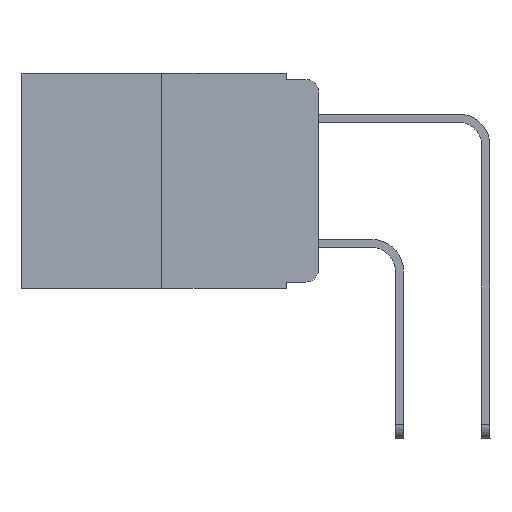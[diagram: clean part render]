
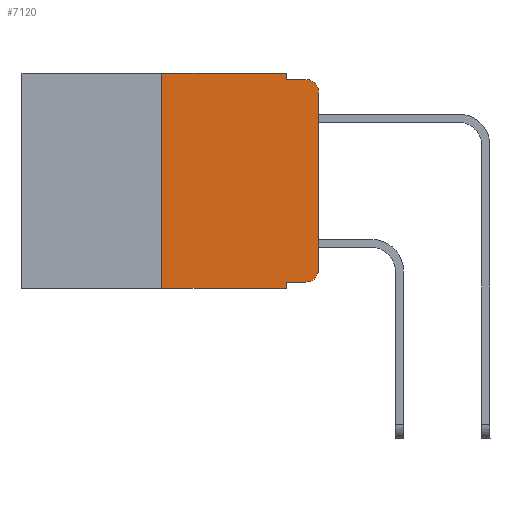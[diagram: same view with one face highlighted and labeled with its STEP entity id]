
A CAD part, left-side view. The second image highlights one B-rep face of the part: STEP entity #7120.
In plain terms, the highlighted planar face has unit normal (-1, 0, 0).
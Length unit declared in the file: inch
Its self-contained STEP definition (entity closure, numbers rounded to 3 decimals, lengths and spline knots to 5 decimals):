
#193 = CARTESIAN_POINT ( 'NONE',  ( 0., 0.473, 0. ) ) ;
#312 = VERTEX_POINT ( 'NONE', #9837 ) ;
#539 = ORIENTED_EDGE ( 'NONE', *, *, #7742, .F. ) ;
#586 = VECTOR ( 'NONE', #9702, 39.37008 ) ;
#711 = CARTESIAN_POINT ( 'NONE',  ( 0., 0.25, -0.343 ) ) ;
#845 = DIRECTION ( 'NONE',  ( 0., 0., -1. ) ) ;
#947 = LINE ( 'NONE', #4866, #586 ) ;
#954 = EDGE_CURVE ( 'NONE', #5619, #1079, #7166, .T. ) ;
#1079 = VERTEX_POINT ( 'NONE', #5046 ) ;
#1091 = EDGE_CURVE ( 'NONE', #1547, #6179, #9170, .T. ) ;
#1263 = CARTESIAN_POINT ( 'NONE',  ( 0., 0.051, -0.343 ) ) ;
#1268 = CARTESIAN_POINT ( 'NONE',  ( 0., 0.02, -0.313 ) ) ;
#1378 = EDGE_CURVE ( 'NONE', #1547, #5619, #9984, .T. ) ;
#1421 = ORIENTED_EDGE ( 'NONE', *, *, #8279, .F. ) ;
#1547 = VERTEX_POINT ( 'NONE', #9796 ) ;
#2402 = CARTESIAN_POINT ( 'NONE',  ( 0., 0.473, 0. ) ) ;
#2510 = VECTOR ( 'NONE', #5384, 39.37008 ) ;
#2611 = VECTOR ( 'NONE', #11231, 39.37008 ) ;
#2626 = AXIS2_PLACEMENT_3D ( 'NONE', #1268, #9910, #845 ) ;
#2719 = AXIS2_PLACEMENT_3D ( 'NONE', #193, #10028, #5282 ) ;
#2840 = DIRECTION ( 'NONE',  ( 0., -1., 0. ) ) ;
#2870 = VERTEX_POINT ( 'NONE', #3173 ) ;
#2975 = VECTOR ( 'NONE', #2840, 39.37008 ) ;
#3173 = CARTESIAN_POINT ( 'NONE',  ( 0., 0.051, 0. ) ) ;
#3471 = VECTOR ( 'NONE', #6111, 39.37008 ) ;
#3953 = ORIENTED_EDGE ( 'NONE', *, *, #1091, .F. ) ;
#4580 = EDGE_LOOP ( 'NONE', ( #8659, #5937, #6307, #1421, #7128, #539, #10409, #3953, #6541, #10649 ) ) ;
#4604 = FACE_OUTER_BOUND ( 'NONE', #4580, .T. ) ;
#4866 = CARTESIAN_POINT ( 'NONE',  ( 0., 0.473, -0.343 ) ) ;
#4942 = CARTESIAN_POINT ( 'NONE',  ( 0., 0., -0.03 ) ) ;
#5011 = VECTOR ( 'NONE', #6856, 39.37008 ) ;
#5046 = CARTESIAN_POINT ( 'NONE',  ( 0., 0., -0.313 ) ) ;
#5282 = DIRECTION ( 'NONE',  ( 0., 0., -1. ) ) ;
#5384 = DIRECTION ( 'NONE',  ( 0., 0., 1. ) ) ;
#5436 = LINE ( 'NONE', #10286, #2975 ) ;
#5619 = VERTEX_POINT ( 'NONE', #10548 ) ;
#5700 = CARTESIAN_POINT ( 'NONE',  ( 0., 0., 0. ) ) ;
#5864 = LINE ( 'NONE', #2402, #3471 ) ;
#5914 = DIRECTION ( 'NONE',  ( -1., 0., 0. ) ) ;
#5937 = ORIENTED_EDGE ( 'NONE', *, *, #9814, .T. ) ;
#5978 = CARTESIAN_POINT ( 'NONE',  ( 0., 0.051, -0.01 ) ) ;
#6111 = DIRECTION ( 'NONE',  ( 0., -1., 0. ) ) ;
#6179 = VERTEX_POINT ( 'NONE', #1263 ) ;
#6307 = ORIENTED_EDGE ( 'NONE', *, *, #8779, .F. ) ;
#6508 = DIRECTION ( 'NONE',  ( 0., 0., 1. ) ) ;
#6541 = ORIENTED_EDGE ( 'NONE', *, *, #1378, .T. ) ;
#6646 = EDGE_CURVE ( 'NONE', #1079, #9744, #6838, .T. ) ;
#6838 = LINE ( 'NONE', #5700, #10460 ) ;
#6856 = DIRECTION ( 'NONE',  ( 0., 0., -1. ) ) ;
#7120 = ADVANCED_FACE ( 'NONE', ( #4604 ), #8495, .F. ) ;
#7128 = ORIENTED_EDGE ( 'NONE', *, *, #7620, .F. ) ;
#7166 = CIRCLE ( 'NONE', #2626, 0.02 ) ;
#7620 = EDGE_CURVE ( 'NONE', #9945, #2870, #5864, .T. ) ;
#7742 = EDGE_CURVE ( 'NONE', #8850, #9945, #11265, .T. ) ;
#7835 = CARTESIAN_POINT ( 'NONE',  ( 0., 0.25, 0. ) ) ;
#7937 = VECTOR ( 'NONE', #10841, 39.37008 ) ;
#8050 = CARTESIAN_POINT ( 'NONE',  ( 0., 0.25, 0. ) ) ;
#8279 = EDGE_CURVE ( 'NONE', #2870, #10180, #9327, .T. ) ;
#8495 = PLANE ( 'NONE',  #2719 ) ;
#8659 = ORIENTED_EDGE ( 'NONE', *, *, #6646, .T. ) ;
#8779 = EDGE_CURVE ( 'NONE', #10180, #312, #5436, .T. ) ;
#8850 = VERTEX_POINT ( 'NONE', #711 ) ;
#9170 = LINE ( 'NONE', #10195, #2611 ) ;
#9327 = LINE ( 'NONE', #9983, #5011 ) ;
#9654 = EDGE_CURVE ( 'NONE', #8850, #6179, #947, .T. ) ;
#9702 = DIRECTION ( 'NONE',  ( 0., -1., 0. ) ) ;
#9744 = VERTEX_POINT ( 'NONE', #4942 ) ;
#9796 = CARTESIAN_POINT ( 'NONE',  ( 0., 0.051, -0.333 ) ) ;
#9814 = EDGE_CURVE ( 'NONE', #9744, #312, #11234, .T. ) ;
#9837 = CARTESIAN_POINT ( 'NONE',  ( 0., 0.02, -0.01 ) ) ;
#9910 = DIRECTION ( 'NONE',  ( -1., 0., 0. ) ) ;
#9945 = VERTEX_POINT ( 'NONE', #8050 ) ;
#9983 = CARTESIAN_POINT ( 'NONE',  ( 0., 0.051, 0. ) ) ;
#9984 = LINE ( 'NONE', #10881, #7937 ) ;
#10028 = DIRECTION ( 'NONE',  ( 1., 0., 0. ) ) ;
#10180 = VERTEX_POINT ( 'NONE', #5978 ) ;
#10195 = CARTESIAN_POINT ( 'NONE',  ( 0., 0.051, 0. ) ) ;
#10286 = CARTESIAN_POINT ( 'NONE',  ( 0., 0.051, -0.01 ) ) ;
#10348 = AXIS2_PLACEMENT_3D ( 'NONE', #10542, #5914, #11280 ) ;
#10409 = ORIENTED_EDGE ( 'NONE', *, *, #9654, .T. ) ;
#10460 = VECTOR ( 'NONE', #6508, 39.37008 ) ;
#10542 = CARTESIAN_POINT ( 'NONE',  ( 0., 0.02, -0.03 ) ) ;
#10548 = CARTESIAN_POINT ( 'NONE',  ( 0., 0.02, -0.333 ) ) ;
#10649 = ORIENTED_EDGE ( 'NONE', *, *, #954, .T. ) ;
#10841 = DIRECTION ( 'NONE',  ( 0., -1., 0. ) ) ;
#10881 = CARTESIAN_POINT ( 'NONE',  ( 0., 0.051, -0.333 ) ) ;
#11231 = DIRECTION ( 'NONE',  ( 0., 0., -1. ) ) ;
#11234 = CIRCLE ( 'NONE', #10348, 0.02 ) ;
#11265 = LINE ( 'NONE', #7835, #2510 ) ;
#11280 = DIRECTION ( 'NONE',  ( 0., 0., -1. ) ) ;
